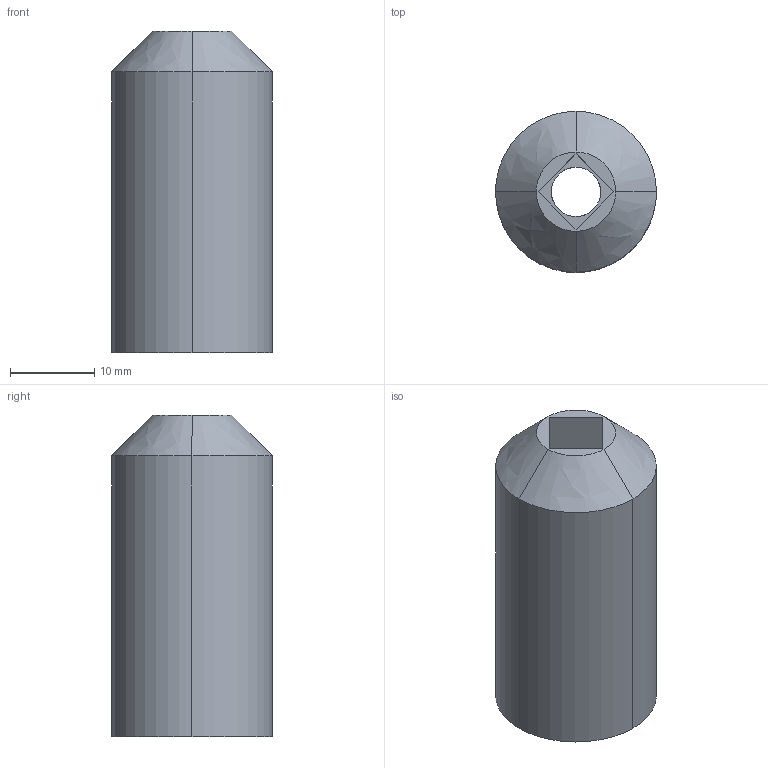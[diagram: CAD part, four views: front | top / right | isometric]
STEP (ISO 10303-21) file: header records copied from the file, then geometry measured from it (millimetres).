
FILE_DESCRIPTION(('Open CASCADE Model'),'2;1');
FILE_NAME('Open CASCADE Shape Model','2013-06-16T13:44:30',('Author'),( 'Open CASCADE'),'Open CASCADE STEP processor 6.1','Open CASCADE 6.1' ,'Unknown');
FILE_SCHEMA(('AUTOMOTIVE_DESIGN_CC2 { 1 2 10303 214 -1 1 5 4 }'));
Length unit declared in the file: millimetre
Products named in the file (1): Product 1
Bounding box: 19.05 x 19.05 x 38.1 mm (x, y, z)
Volume: 7311.5 mm3; surface area: 3768.9 mm2
Topology: 1 solids, 1 shells, 24 faces, 56 edges, 36 vertices
Faces by surface type: bspline 20, plane 4
Entity records: 4922 total; most frequent: CARTESIAN_POINT 4033, ORIENTED_EDGE 112, PCURVE 112, DEFINITIONAL_REPRESENTATION 112, DIRECTION 86, B_SPLINE_CURVE_WITH_KNOTS 68, LINE 64, VECTOR 64
